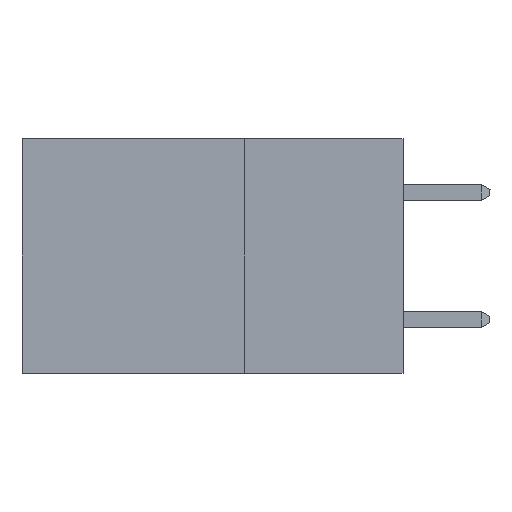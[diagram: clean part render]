
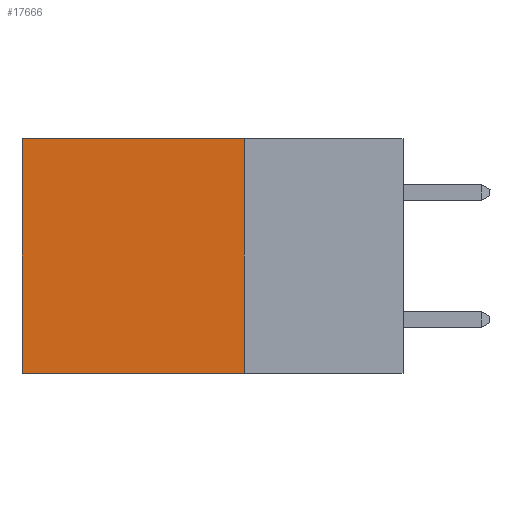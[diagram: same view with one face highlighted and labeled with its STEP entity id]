
A CAD part, left-side view. The second image highlights one B-rep face of the part: STEP entity #17666.
In plain terms, the highlighted planar face has unit normal (-1, 0, 0).
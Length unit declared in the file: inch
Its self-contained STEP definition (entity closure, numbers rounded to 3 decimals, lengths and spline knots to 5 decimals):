
#70 = DIRECTION ( 'NONE',  ( 1., 0., 0. ) ) ;
#220 = VECTOR ( 'NONE', #10149, 39.37008 ) ;
#704 = VERTEX_POINT ( 'NONE', #14856 ) ;
#1668 = CARTESIAN_POINT ( 'NONE',  ( 0.2875, 0.25, 0. ) ) ;
#1778 = LINE ( 'NONE', #8307, #220 ) ;
#1939 = DIRECTION ( 'NONE',  ( 0., 0., -1. ) ) ;
#2604 = ORIENTED_EDGE ( 'NONE', *, *, #20254, .F. ) ;
#2717 = ORIENTED_EDGE ( 'NONE', *, *, #7263, .T. ) ;
#3514 = PLANE ( 'NONE',  #7288 ) ;
#3973 = CARTESIAN_POINT ( 'NONE',  ( 0.2875, 0.6, 0. ) ) ;
#4568 = ORIENTED_EDGE ( 'NONE', *, *, #5966, .T. ) ;
#4660 = LINE ( 'NONE', #5320, #20992 ) ;
#5320 = CARTESIAN_POINT ( 'NONE',  ( 0.2875, 0.25, 0. ) ) ;
#5966 = EDGE_CURVE ( 'NONE', #8487, #8129, #4660, .T. ) ;
#6472 = ORIENTED_EDGE ( 'NONE', *, *, #11447, .F. ) ;
#6683 = CARTESIAN_POINT ( 'NONE',  ( 0.2875, 0.25, -0.37 ) ) ;
#7263 = EDGE_CURVE ( 'NONE', #8129, #15154, #1778, .T. ) ;
#7288 = AXIS2_PLACEMENT_3D ( 'NONE', #16556, #70, #1939 ) ;
#8068 = LINE ( 'NONE', #10897, #17492 ) ;
#8129 = VERTEX_POINT ( 'NONE', #3973 ) ;
#8307 = CARTESIAN_POINT ( 'NONE',  ( 0.2875, 0.6, 0. ) ) ;
#8487 = VERTEX_POINT ( 'NONE', #1668 ) ;
#9806 = EDGE_LOOP ( 'NONE', ( #2717, #6472, #2604, #4568 ) ) ;
#10149 = DIRECTION ( 'NONE',  ( 0., 0., -1. ) ) ;
#10241 = DIRECTION ( 'NONE',  ( 0., 1., 0. ) ) ;
#10807 = FACE_OUTER_BOUND ( 'NONE', #9806, .T. ) ;
#10897 = CARTESIAN_POINT ( 'NONE',  ( 0.2875, 0.25, 0. ) ) ;
#11447 = EDGE_CURVE ( 'NONE', #704, #15154, #13194, .T. ) ;
#11909 = VECTOR ( 'NONE', #10241, 39.37008 ) ;
#12029 = CARTESIAN_POINT ( 'NONE',  ( 0.2875, 0.6, -0.37 ) ) ;
#13194 = LINE ( 'NONE', #6683, #11909 ) ;
#14856 = CARTESIAN_POINT ( 'NONE',  ( 0.2875, 0.25, -0.37 ) ) ;
#15154 = VERTEX_POINT ( 'NONE', #12029 ) ;
#16556 = CARTESIAN_POINT ( 'NONE',  ( 0.2875, 0.25, 0. ) ) ;
#16702 = DIRECTION ( 'NONE',  ( 0., 1., 0. ) ) ;
#17378 = DIRECTION ( 'NONE',  ( 0., 0., -1. ) ) ;
#17492 = VECTOR ( 'NONE', #17378, 39.37008 ) ;
#17666 = ADVANCED_FACE ( 'NONE', ( #10807 ), #3514, .F. ) ;
#20254 = EDGE_CURVE ( 'NONE', #8487, #704, #8068, .T. ) ;
#20992 = VECTOR ( 'NONE', #16702, 39.37008 ) ;
